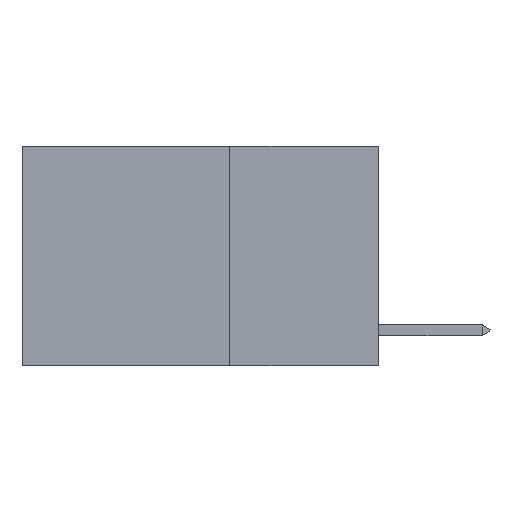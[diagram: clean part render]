
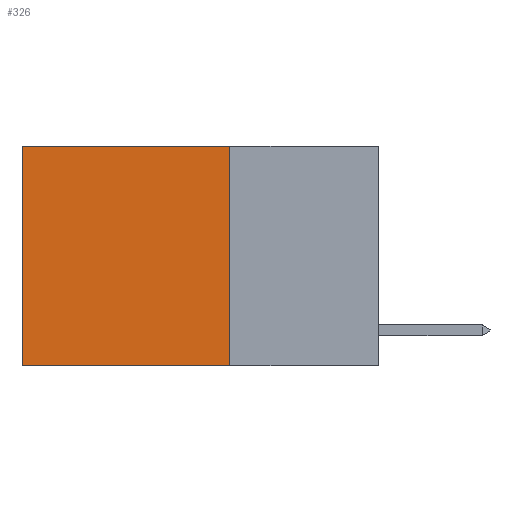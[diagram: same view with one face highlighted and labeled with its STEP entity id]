
A CAD part, left-side view. The second image highlights one B-rep face of the part: STEP entity #326.
In plain terms, the highlighted planar face has unit normal (-1, 0, 0).
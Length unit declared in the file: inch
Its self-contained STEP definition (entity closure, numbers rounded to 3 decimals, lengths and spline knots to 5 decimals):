
#54 = CARTESIAN_POINT ( 'NONE',  ( 0.2625, 0.25, 0. ) ) ;
#326 = ADVANCED_FACE ( 'NONE', ( #13382 ), #1222, .F. ) ;
#1027 = VECTOR ( 'NONE', #10893, 39.37008 ) ;
#1222 = PLANE ( 'NONE',  #10810 ) ;
#1927 = ORIENTED_EDGE ( 'NONE', *, *, #19322, .T. ) ;
#2155 = EDGE_CURVE ( 'NONE', #13999, #21222, #12219, .T. ) ;
#3474 = ORIENTED_EDGE ( 'NONE', *, *, #2155, .F. ) ;
#3980 = DIRECTION ( 'NONE',  ( 0., 0., -1. ) ) ;
#5133 = ORIENTED_EDGE ( 'NONE', *, *, #10625, .T. ) ;
#5821 = CARTESIAN_POINT ( 'NONE',  ( 0.2625, 0.6, 0. ) ) ;
#6403 = CARTESIAN_POINT ( 'NONE',  ( 0.2625, 0.6, 0. ) ) ;
#6415 = DIRECTION ( 'NONE',  ( 0., 0., -1. ) ) ;
#7090 = CARTESIAN_POINT ( 'NONE',  ( 0.2625, 0.25, -0.37 ) ) ;
#7137 = ORIENTED_EDGE ( 'NONE', *, *, #21997, .F. ) ;
#7264 = CARTESIAN_POINT ( 'NONE',  ( 0.2625, 0.25, 0. ) ) ;
#8309 = CARTESIAN_POINT ( 'NONE',  ( 0.2625, 0.25, 0. ) ) ;
#8456 = VECTOR ( 'NONE', #12102, 39.37008 ) ;
#9187 = LINE ( 'NONE', #54, #8456 ) ;
#9555 = DIRECTION ( 'NONE',  ( 0., 0., -1. ) ) ;
#10625 = EDGE_CURVE ( 'NONE', #20583, #21222, #21788, .T. ) ;
#10810 = AXIS2_PLACEMENT_3D ( 'NONE', #8309, #20108, #6415 ) ;
#10893 = DIRECTION ( 'NONE',  ( 0., 1., 0. ) ) ;
#11538 = VECTOR ( 'NONE', #9555, 39.37008 ) ;
#12102 = DIRECTION ( 'NONE',  ( 0., 1., 0. ) ) ;
#12219 = LINE ( 'NONE', #7090, #1027 ) ;
#13030 = CARTESIAN_POINT ( 'NONE',  ( 0.2625, 0.25, -0.37 ) ) ;
#13211 = VECTOR ( 'NONE', #3980, 39.37008 ) ;
#13382 = FACE_OUTER_BOUND ( 'NONE', #14937, .T. ) ;
#13999 = VERTEX_POINT ( 'NONE', #13030 ) ;
#14168 = VERTEX_POINT ( 'NONE', #20549 ) ;
#14937 = EDGE_LOOP ( 'NONE', ( #5133, #3474, #7137, #1927 ) ) ;
#17826 = LINE ( 'NONE', #7264, #13211 ) ;
#19322 = EDGE_CURVE ( 'NONE', #14168, #20583, #9187, .T. ) ;
#19941 = CARTESIAN_POINT ( 'NONE',  ( 0.2625, 0.6, -0.37 ) ) ;
#20108 = DIRECTION ( 'NONE',  ( 1., 0., 0. ) ) ;
#20549 = CARTESIAN_POINT ( 'NONE',  ( 0.2625, 0.25, 0. ) ) ;
#20583 = VERTEX_POINT ( 'NONE', #5821 ) ;
#21222 = VERTEX_POINT ( 'NONE', #19941 ) ;
#21788 = LINE ( 'NONE', #6403, #11538 ) ;
#21997 = EDGE_CURVE ( 'NONE', #14168, #13999, #17826, .T. ) ;
